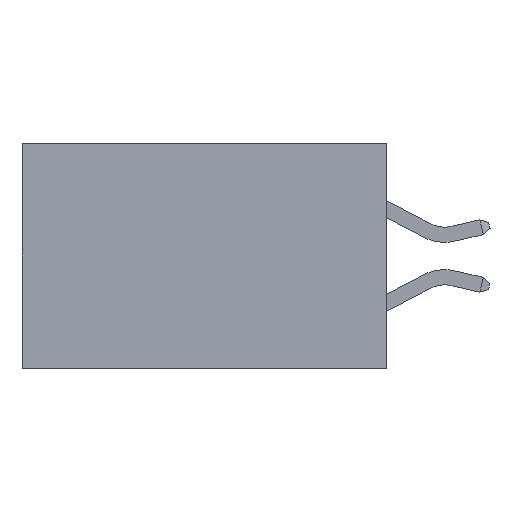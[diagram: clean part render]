
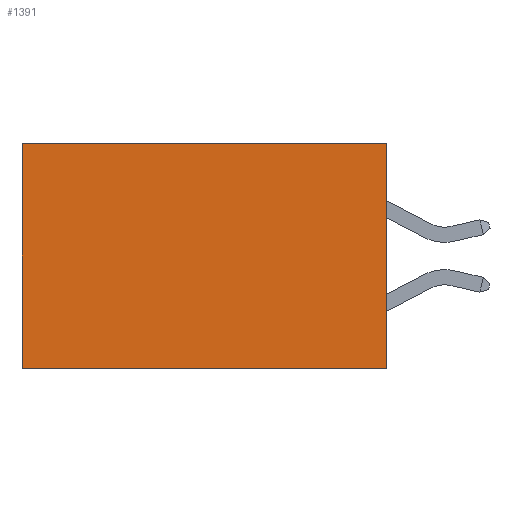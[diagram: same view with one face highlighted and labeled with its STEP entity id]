
A CAD part, left-side view. The second image highlights one B-rep face of the part: STEP entity #1391.
In plain terms, the highlighted planar face has unit normal (-1, 0, 0).
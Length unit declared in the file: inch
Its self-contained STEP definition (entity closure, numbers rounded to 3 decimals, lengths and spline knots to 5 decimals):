
#312 = DIRECTION ( 'NONE',  ( 0., 0., -1. ) ) ;
#1362 = VERTEX_POINT ( 'NONE', #15029 ) ;
#1391 = ADVANCED_FACE ( 'NONE', ( #22237 ), #11157, .F. ) ;
#2083 = DIRECTION ( 'NONE',  ( 0., 1., 0. ) ) ;
#2296 = AXIS2_PLACEMENT_3D ( 'NONE', #21239, #23106, #6072 ) ;
#3472 = LINE ( 'NONE', #23132, #16979 ) ;
#3755 = VECTOR ( 'NONE', #11693, 39.37008 ) ;
#4291 = VERTEX_POINT ( 'NONE', #7142 ) ;
#4304 = LINE ( 'NONE', #15495, #11813 ) ;
#4721 = VERTEX_POINT ( 'NONE', #16116 ) ;
#5255 = EDGE_CURVE ( 'NONE', #24316, #4721, #4304, .T. ) ;
#5259 = EDGE_CURVE ( 'NONE', #4291, #4721, #12730, .T. ) ;
#6072 = DIRECTION ( 'NONE',  ( 0., 0., -1. ) ) ;
#6252 = CARTESIAN_POINT ( 'NONE',  ( 0.298, 0., 0. ) ) ;
#7142 = CARTESIAN_POINT ( 'NONE',  ( 0.298, 0.6, 0. ) ) ;
#8052 = ORIENTED_EDGE ( 'NONE', *, *, #12245, .T. ) ;
#8723 = ORIENTED_EDGE ( 'NONE', *, *, #5259, .T. ) ;
#9816 = CARTESIAN_POINT ( 'NONE',  ( 0.298, 0., -0.37 ) ) ;
#11157 = PLANE ( 'NONE',  #2296 ) ;
#11693 = DIRECTION ( 'NONE',  ( 0., 0., -1. ) ) ;
#11813 = VECTOR ( 'NONE', #2083, 39.37008 ) ;
#12119 = VECTOR ( 'NONE', #312, 39.37008 ) ;
#12245 = EDGE_CURVE ( 'NONE', #1362, #4291, #3472, .T. ) ;
#12730 = LINE ( 'NONE', #23314, #12119 ) ;
#13548 = DIRECTION ( 'NONE',  ( 0., 1., 0. ) ) ;
#13976 = LINE ( 'NONE', #6252, #3755 ) ;
#14324 = ORIENTED_EDGE ( 'NONE', *, *, #22262, .F. ) ;
#15029 = CARTESIAN_POINT ( 'NONE',  ( 0.298, 0., 0. ) ) ;
#15495 = CARTESIAN_POINT ( 'NONE',  ( 0.298, 0., -0.37 ) ) ;
#16116 = CARTESIAN_POINT ( 'NONE',  ( 0.298, 0.6, -0.37 ) ) ;
#16979 = VECTOR ( 'NONE', #13548, 39.37008 ) ;
#21239 = CARTESIAN_POINT ( 'NONE',  ( 0.298, 0., 0. ) ) ;
#22237 = FACE_OUTER_BOUND ( 'NONE', #23562, .T. ) ;
#22262 = EDGE_CURVE ( 'NONE', #1362, #24316, #13976, .T. ) ;
#23106 = DIRECTION ( 'NONE',  ( 1., 0., 0. ) ) ;
#23132 = CARTESIAN_POINT ( 'NONE',  ( 0.298, 0., 0. ) ) ;
#23172 = ORIENTED_EDGE ( 'NONE', *, *, #5255, .F. ) ;
#23314 = CARTESIAN_POINT ( 'NONE',  ( 0.298, 0.6, 0. ) ) ;
#23562 = EDGE_LOOP ( 'NONE', ( #8723, #23172, #14324, #8052 ) ) ;
#24316 = VERTEX_POINT ( 'NONE', #9816 ) ;
